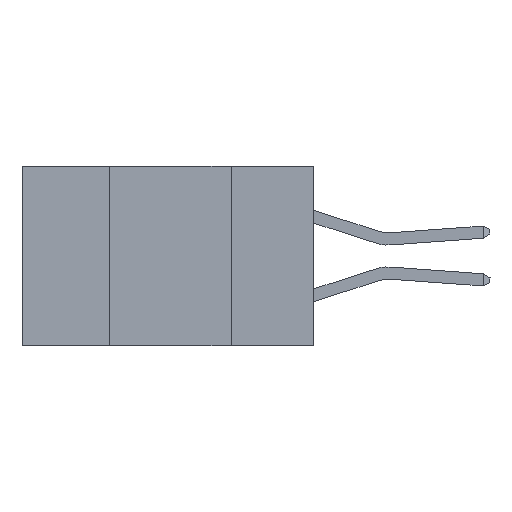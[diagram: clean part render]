
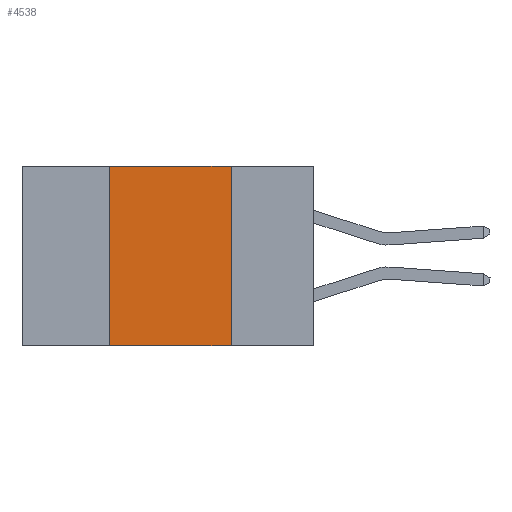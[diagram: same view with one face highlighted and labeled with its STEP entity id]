
A CAD part, left-side view. The second image highlights one B-rep face of the part: STEP entity #4538.
In plain terms, the highlighted planar face has unit normal (-1, 0, 0).
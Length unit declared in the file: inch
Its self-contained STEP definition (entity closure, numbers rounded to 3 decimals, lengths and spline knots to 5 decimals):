
#818 = ORIENTED_EDGE ( 'NONE', *, *, #9055, .F. ) ;
#1195 = ORIENTED_EDGE ( 'NONE', *, *, #13598, .T. ) ;
#1632 = VERTEX_POINT ( 'NONE', #17392 ) ;
#1989 = ORIENTED_EDGE ( 'NONE', *, *, #12548, .F. ) ;
#2507 = VECTOR ( 'NONE', #15274, 39.37008 ) ;
#2603 = CARTESIAN_POINT ( 'NONE',  ( 0., 0.42, 0. ) ) ;
#2785 = LINE ( 'NONE', #16939, #5662 ) ;
#3315 = LINE ( 'NONE', #6468, #13647 ) ;
#3881 = EDGE_LOOP ( 'NONE', ( #1989, #10596, #818, #1195 ) ) ;
#3902 = VERTEX_POINT ( 'NONE', #4191 ) ;
#4191 = CARTESIAN_POINT ( 'NONE',  ( 0., 0.17, -0.37 ) ) ;
#4538 = ADVANCED_FACE ( 'NONE', ( #13711 ), #11107, .F. ) ;
#4850 = LINE ( 'NONE', #2603, #14264 ) ;
#4920 = VERTEX_POINT ( 'NONE', #6817 ) ;
#5662 = VECTOR ( 'NONE', #13043, 39.37008 ) ;
#6468 = CARTESIAN_POINT ( 'NONE',  ( 0., 0.6, 0. ) ) ;
#6677 = LINE ( 'NONE', #8682, #2507 ) ;
#6817 = CARTESIAN_POINT ( 'NONE',  ( 0., 0.17, 0. ) ) ;
#6885 = DIRECTION ( 'NONE',  ( 0., 0., 1. ) ) ;
#6899 = CARTESIAN_POINT ( 'NONE',  ( 0., 0.42, 0. ) ) ;
#7895 = DIRECTION ( 'NONE',  ( 0., -1., 0. ) ) ;
#8682 = CARTESIAN_POINT ( 'NONE',  ( 0., 0.6, -0.37 ) ) ;
#8882 = EDGE_CURVE ( 'NONE', #10391, #4920, #3315, .T. ) ;
#9055 = EDGE_CURVE ( 'NONE', #1632, #10391, #4850, .T. ) ;
#10391 = VERTEX_POINT ( 'NONE', #6899 ) ;
#10596 = ORIENTED_EDGE ( 'NONE', *, *, #8882, .F. ) ;
#11047 = DIRECTION ( 'NONE',  ( 0., 0., -1. ) ) ;
#11064 = DIRECTION ( 'NONE',  ( 1., 0., 0. ) ) ;
#11107 = PLANE ( 'NONE',  #14418 ) ;
#11147 = CARTESIAN_POINT ( 'NONE',  ( 0., 0.6, 0. ) ) ;
#12548 = EDGE_CURVE ( 'NONE', #4920, #3902, #2785, .T. ) ;
#13043 = DIRECTION ( 'NONE',  ( 0., 0., -1. ) ) ;
#13598 = EDGE_CURVE ( 'NONE', #1632, #3902, #6677, .T. ) ;
#13647 = VECTOR ( 'NONE', #7895, 39.37008 ) ;
#13711 = FACE_OUTER_BOUND ( 'NONE', #3881, .T. ) ;
#14264 = VECTOR ( 'NONE', #6885, 39.37008 ) ;
#14418 = AXIS2_PLACEMENT_3D ( 'NONE', #11147, #11064, #11047 ) ;
#15274 = DIRECTION ( 'NONE',  ( 0., -1., 0. ) ) ;
#16939 = CARTESIAN_POINT ( 'NONE',  ( 0., 0.17, 0. ) ) ;
#17392 = CARTESIAN_POINT ( 'NONE',  ( 0., 0.42, -0.37 ) ) ;
